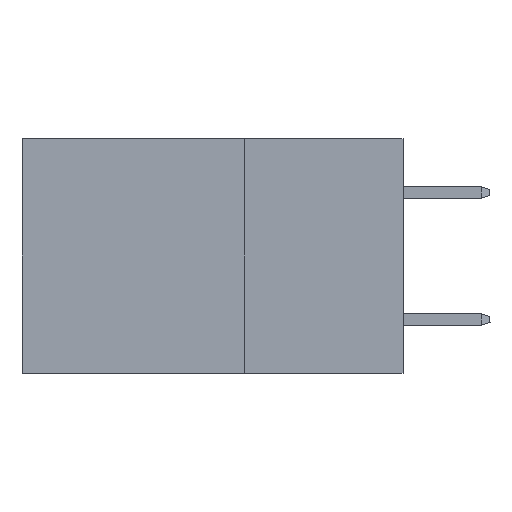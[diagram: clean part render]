
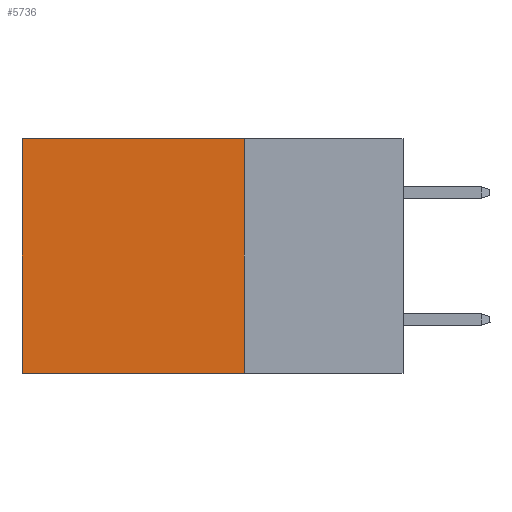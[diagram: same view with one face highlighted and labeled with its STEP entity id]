
A CAD part, left-side view. The second image highlights one B-rep face of the part: STEP entity #5736.
In plain terms, the highlighted planar face has unit normal (-1, 0, 0).
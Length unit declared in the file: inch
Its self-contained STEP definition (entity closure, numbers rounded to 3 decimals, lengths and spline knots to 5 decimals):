
#29 = VECTOR ( 'NONE', #14733, 39.37008 ) ;
#76 = VERTEX_POINT ( 'NONE', #14246 ) ;
#446 = CARTESIAN_POINT ( 'NONE',  ( 0.2875, 0.25, -0.37 ) ) ;
#1605 = CARTESIAN_POINT ( 'NONE',  ( 0.2875, 0.25, 0. ) ) ;
#1878 = CARTESIAN_POINT ( 'NONE',  ( 0.2875, 0.25, -0.37 ) ) ;
#2650 = DIRECTION ( 'NONE',  ( 0., 0., -1. ) ) ;
#2888 = AXIS2_PLACEMENT_3D ( 'NONE', #9300, #21010, #2650 ) ;
#3072 = VERTEX_POINT ( 'NONE', #1878 ) ;
#4144 = EDGE_LOOP ( 'NONE', ( #12523, #19062, #15524, #15516 ) ) ;
#5456 = LINE ( 'NONE', #446, #13795 ) ;
#5736 = ADVANCED_FACE ( 'NONE', ( #19451 ), #17764, .F. ) ;
#6229 = EDGE_CURVE ( 'NONE', #14999, #76, #11056, .T. ) ;
#7798 = VECTOR ( 'NONE', #7835, 39.37008 ) ;
#7835 = DIRECTION ( 'NONE',  ( 0., 0., -1. ) ) ;
#9300 = CARTESIAN_POINT ( 'NONE',  ( 0.2875, 0.25, 0. ) ) ;
#10238 = DIRECTION ( 'NONE',  ( 0., 1., 0. ) ) ;
#11056 = LINE ( 'NONE', #14284, #16619 ) ;
#11148 = EDGE_CURVE ( 'NONE', #76, #15032, #18317, .T. ) ;
#12523 = ORIENTED_EDGE ( 'NONE', *, *, #11148, .T. ) ;
#13422 = CARTESIAN_POINT ( 'NONE',  ( 0.2875, 0.6, -0.37 ) ) ;
#13795 = VECTOR ( 'NONE', #10238, 39.37008 ) ;
#14246 = CARTESIAN_POINT ( 'NONE',  ( 0.2875, 0.6, 0. ) ) ;
#14284 = CARTESIAN_POINT ( 'NONE',  ( 0.2875, 0.25, 0. ) ) ;
#14289 = EDGE_CURVE ( 'NONE', #14999, #3072, #19854, .T. ) ;
#14733 = DIRECTION ( 'NONE',  ( 0., 0., -1. ) ) ;
#14999 = VERTEX_POINT ( 'NONE', #20219 ) ;
#15032 = VERTEX_POINT ( 'NONE', #13422 ) ;
#15516 = ORIENTED_EDGE ( 'NONE', *, *, #6229, .T. ) ;
#15524 = ORIENTED_EDGE ( 'NONE', *, *, #14289, .F. ) ;
#16074 = EDGE_CURVE ( 'NONE', #3072, #15032, #5456, .T. ) ;
#16619 = VECTOR ( 'NONE', #21094, 39.37008 ) ;
#17764 = PLANE ( 'NONE',  #2888 ) ;
#18317 = LINE ( 'NONE', #21325, #7798 ) ;
#19062 = ORIENTED_EDGE ( 'NONE', *, *, #16074, .F. ) ;
#19451 = FACE_OUTER_BOUND ( 'NONE', #4144, .T. ) ;
#19854 = LINE ( 'NONE', #1605, #29 ) ;
#20219 = CARTESIAN_POINT ( 'NONE',  ( 0.2875, 0.25, 0. ) ) ;
#21010 = DIRECTION ( 'NONE',  ( 1., 0., 0. ) ) ;
#21094 = DIRECTION ( 'NONE',  ( 0., 1., 0. ) ) ;
#21325 = CARTESIAN_POINT ( 'NONE',  ( 0.2875, 0.6, 0. ) ) ;
